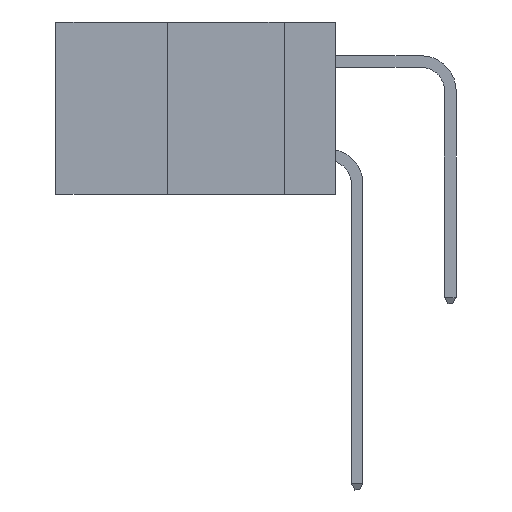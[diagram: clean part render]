
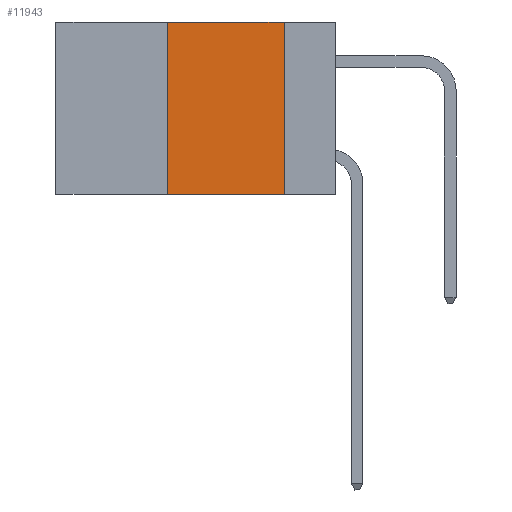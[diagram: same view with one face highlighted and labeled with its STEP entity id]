
A CAD part, left-side view. The second image highlights one B-rep face of the part: STEP entity #11943.
In plain terms, the highlighted planar face has unit normal (-1, 0, 0).
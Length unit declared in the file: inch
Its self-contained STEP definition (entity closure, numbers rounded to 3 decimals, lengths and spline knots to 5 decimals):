
#882 = CARTESIAN_POINT ( 'NONE',  ( 0., 0.11, 0. ) ) ;
#1428 = EDGE_LOOP ( 'NONE', ( #5949, #12743, #16313, #6792 ) ) ;
#2174 = VERTEX_POINT ( 'NONE', #6153 ) ;
#2943 = CARTESIAN_POINT ( 'NONE',  ( 0., 0.6, 0. ) ) ;
#4139 = VECTOR ( 'NONE', #15602, 39.37008 ) ;
#4251 = DIRECTION ( 'NONE',  ( 0., 0., -1. ) ) ;
#4478 = EDGE_CURVE ( 'NONE', #15363, #2174, #13897, .T. ) ;
#4494 = CARTESIAN_POINT ( 'NONE',  ( 0., 0.36, 0. ) ) ;
#5551 = CARTESIAN_POINT ( 'NONE',  ( 0., 0.6, -0.37 ) ) ;
#5609 = DIRECTION ( 'NONE',  ( 0., 0., -1. ) ) ;
#5949 = ORIENTED_EDGE ( 'NONE', *, *, #4478, .F. ) ;
#6153 = CARTESIAN_POINT ( 'NONE',  ( 0., 0.11, -0.37 ) ) ;
#6156 = VERTEX_POINT ( 'NONE', #6275 ) ;
#6275 = CARTESIAN_POINT ( 'NONE',  ( 0., 0.36, -0.37 ) ) ;
#6449 = VERTEX_POINT ( 'NONE', #16243 ) ;
#6476 = VECTOR ( 'NONE', #8487, 39.37008 ) ;
#6792 = ORIENTED_EDGE ( 'NONE', *, *, #12547, .T. ) ;
#7020 = CARTESIAN_POINT ( 'NONE',  ( 0., 0.11, 0. ) ) ;
#7035 = AXIS2_PLACEMENT_3D ( 'NONE', #2943, #11981, #4251 ) ;
#7218 = VECTOR ( 'NONE', #5609, 39.37008 ) ;
#7257 = LINE ( 'NONE', #5551, #4139 ) ;
#8487 = DIRECTION ( 'NONE',  ( 0., 0., 1. ) ) ;
#9571 = LINE ( 'NONE', #4494, #6476 ) ;
#10753 = PLANE ( 'NONE',  #7035 ) ;
#11228 = DIRECTION ( 'NONE',  ( 0., -1., 0. ) ) ;
#11943 = ADVANCED_FACE ( 'NONE', ( #13380 ), #10753, .F. ) ;
#11981 = DIRECTION ( 'NONE',  ( 1., 0., 0. ) ) ;
#12547 = EDGE_CURVE ( 'NONE', #6156, #2174, #7257, .T. ) ;
#12743 = ORIENTED_EDGE ( 'NONE', *, *, #15939, .F. ) ;
#13380 = FACE_OUTER_BOUND ( 'NONE', #1428, .T. ) ;
#13897 = LINE ( 'NONE', #7020, #7218 ) ;
#13952 = LINE ( 'NONE', #16040, #15616 ) ;
#15057 = EDGE_CURVE ( 'NONE', #6156, #6449, #9571, .T. ) ;
#15363 = VERTEX_POINT ( 'NONE', #882 ) ;
#15602 = DIRECTION ( 'NONE',  ( 0., -1., 0. ) ) ;
#15616 = VECTOR ( 'NONE', #11228, 39.37008 ) ;
#15939 = EDGE_CURVE ( 'NONE', #6449, #15363, #13952, .T. ) ;
#16040 = CARTESIAN_POINT ( 'NONE',  ( 0., 0.6, 0. ) ) ;
#16243 = CARTESIAN_POINT ( 'NONE',  ( 0., 0.36, 0. ) ) ;
#16313 = ORIENTED_EDGE ( 'NONE', *, *, #15057, .F. ) ;
